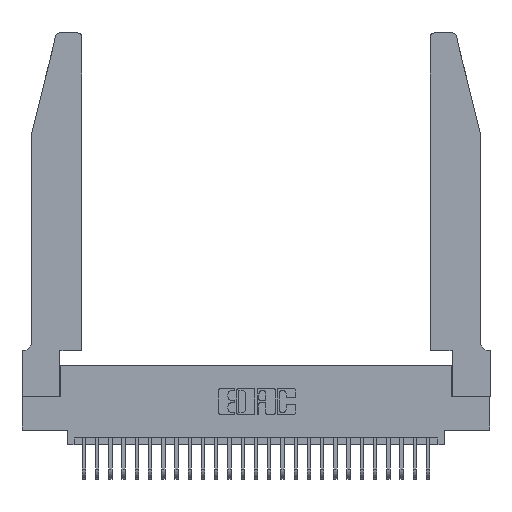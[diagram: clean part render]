
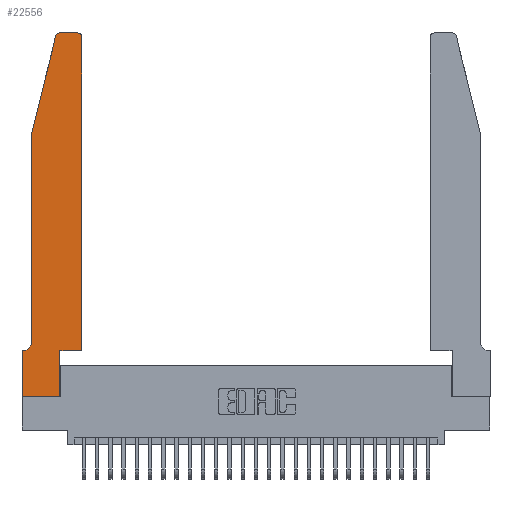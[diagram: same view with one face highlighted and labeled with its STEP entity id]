
A CAD part, top view. The second image highlights one B-rep face of the part: STEP entity #22556.
In plain terms, the highlighted planar face has unit normal (0, 0, 1).
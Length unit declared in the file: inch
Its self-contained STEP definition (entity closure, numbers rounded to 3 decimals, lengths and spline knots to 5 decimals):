
#375 = ORIENTED_EDGE ( 'NONE', *, *, #16951, .T. ) ;
#430 = CARTESIAN_POINT ( 'NONE',  ( 0.4505, 0.35, 0.37 ) ) ;
#533 = ORIENTED_EDGE ( 'NONE', *, *, #11669, .T. ) ;
#1488 = VECTOR ( 'NONE', #29293, 39.37008 ) ;
#1646 = VECTOR ( 'NONE', #20844, 39.37008 ) ;
#1717 = EDGE_CURVE ( 'NONE', #22528, #5723, #22442, .T. ) ;
#1726 = AXIS2_PLACEMENT_3D ( 'NONE', #11985, #23488, #21390 ) ;
#1741 = ORIENTED_EDGE ( 'NONE', *, *, #27079, .T. ) ;
#1800 = CARTESIAN_POINT ( 'NONE',  ( 0., 0., 0.37 ) ) ;
#2905 = CARTESIAN_POINT ( 'NONE',  ( 0.4505, 0.35, 0.37 ) ) ;
#2944 = CARTESIAN_POINT ( 'NONE',  ( 0.0055, 0.35, 0.37 ) ) ;
#3498 = CARTESIAN_POINT ( 'NONE',  ( 0., 0., 0.37 ) ) ;
#3584 = ORIENTED_EDGE ( 'NONE', *, *, #4587, .T. ) ;
#4185 = LINE ( 'NONE', #24555, #15647 ) ;
#4266 = DIRECTION ( 'NONE',  ( -1., 0., 0. ) ) ;
#4587 = EDGE_CURVE ( 'NONE', #23105, #7640, #13670, .T. ) ;
#4947 = CARTESIAN_POINT ( 'NONE',  ( 0.0755, 0.42, 0.37 ) ) ;
#5068 = VERTEX_POINT ( 'NONE', #10028 ) ;
#5439 = VECTOR ( 'NONE', #25315, 39.37008 ) ;
#5459 = ORIENTED_EDGE ( 'NONE', *, *, #1717, .T. ) ;
#5581 = FACE_OUTER_BOUND ( 'NONE', #8684, .T. ) ;
#5723 = VERTEX_POINT ( 'NONE', #19991 ) ;
#6921 = DIRECTION ( 'NONE',  ( 0., -1., 0. ) ) ;
#6987 = ORIENTED_EDGE ( 'NONE', *, *, #10676, .T. ) ;
#7568 = ORIENTED_EDGE ( 'NONE', *, *, #29201, .T. ) ;
#7640 = VERTEX_POINT ( 'NONE', #20944 ) ;
#7680 = CARTESIAN_POINT ( 'NONE',  ( 0.2865, 0.35, 0.37 ) ) ;
#8175 = CARTESIAN_POINT ( 'NONE',  ( 0.4205, 2.75, 0.37 ) ) ;
#8197 = LINE ( 'NONE', #2905, #18227 ) ;
#8434 = LINE ( 'NONE', #11802, #26037 ) ;
#8684 = EDGE_LOOP ( 'NONE', ( #5459, #12279, #17087, #6987, #375, #15100, #533, #3584, #7568, #1741, #19392, #16044 ) ) ;
#9358 = DIRECTION ( 'NONE',  ( 1., 0., 0. ) ) ;
#10028 = CARTESIAN_POINT ( 'NONE',  ( 0.0755, 2., 0.37 ) ) ;
#10676 = EDGE_CURVE ( 'NONE', #5068, #27703, #4185, .T. ) ;
#10767 = CARTESIAN_POINT ( 'NONE',  ( 0.4205, 2.72, 0.37 ) ) ;
#11491 = CARTESIAN_POINT ( 'NONE',  ( 0.4505, 2.72, 0.37 ) ) ;
#11669 = EDGE_CURVE ( 'NONE', #23673, #23105, #23116, .T. ) ;
#11802 = CARTESIAN_POINT ( 'NONE',  ( 0.2865, 0.35, 0.37 ) ) ;
#11940 = DIRECTION ( 'NONE',  ( 0., 0., 1. ) ) ;
#11985 = CARTESIAN_POINT ( 'NONE',  ( 0.0055, 0.42, 0.37 ) ) ;
#12279 = ORIENTED_EDGE ( 'NONE', *, *, #28305, .T. ) ;
#12955 = VECTOR ( 'NONE', #21468, 39.37008 ) ;
#13012 = DIRECTION ( 'NONE',  ( 1., 0., 0. ) ) ;
#13096 = AXIS2_PLACEMENT_3D ( 'NONE', #10767, #27358, #29496 ) ;
#13130 = EDGE_CURVE ( 'NONE', #19596, #28972, #14372, .T. ) ;
#13670 = LINE ( 'NONE', #25472, #12955 ) ;
#14372 = LINE ( 'NONE', #24718, #1488 ) ;
#14900 = DIRECTION ( 'NONE',  ( 0., 0., 1. ) ) ;
#15100 = ORIENTED_EDGE ( 'NONE', *, *, #19973, .T. ) ;
#15647 = VECTOR ( 'NONE', #6921, 39.37008 ) ;
#16044 = ORIENTED_EDGE ( 'NONE', *, *, #19439, .T. ) ;
#16383 = DIRECTION ( 'NONE',  ( 0., 1., 0. ) ) ;
#16781 = CIRCLE ( 'NONE', #13096, 0.03 ) ;
#16951 = EDGE_CURVE ( 'NONE', #27703, #26474, #25640, .T. ) ;
#17087 = ORIENTED_EDGE ( 'NONE', *, *, #24657, .T. ) ;
#17845 = CARTESIAN_POINT ( 'NONE',  ( 0.0755, 0.35, 0.37 ) ) ;
#17927 = LINE ( 'NONE', #22639, #5439 ) ;
#18227 = VECTOR ( 'NONE', #9358, 39.37008 ) ;
#19392 = ORIENTED_EDGE ( 'NONE', *, *, #13130, .T. ) ;
#19439 = EDGE_CURVE ( 'NONE', #28972, #22528, #16781, .T. ) ;
#19596 = VERTEX_POINT ( 'NONE', #430 ) ;
#19973 = EDGE_CURVE ( 'NONE', #26474, #23673, #25398, .T. ) ;
#19991 = CARTESIAN_POINT ( 'NONE',  ( 0.284, 2.75, 0.37 ) ) ;
#20844 = DIRECTION ( 'NONE',  ( -1., 0., 0. ) ) ;
#20944 = CARTESIAN_POINT ( 'NONE',  ( 0.2865, 0., 0.37 ) ) ;
#21280 = AXIS2_PLACEMENT_3D ( 'NONE', #23348, #11940, #21352 ) ;
#21352 = DIRECTION ( 'NONE',  ( 1., 0., 0. ) ) ;
#21390 = DIRECTION ( 'NONE',  ( -1., 0., 0. ) ) ;
#21468 = DIRECTION ( 'NONE',  ( 1., 0., 0. ) ) ;
#22027 = CARTESIAN_POINT ( 'NONE',  ( 0., 0.35, 0.37 ) ) ;
#22442 = LINE ( 'NONE', #23070, #1646 ) ;
#22528 = VERTEX_POINT ( 'NONE', #8175 ) ;
#22556 = ADVANCED_FACE ( 'NONE', ( #5581 ), #24220, .T. ) ;
#22639 = CARTESIAN_POINT ( 'NONE',  ( 0.0755, 2., 0.37 ) ) ;
#23070 = CARTESIAN_POINT ( 'NONE',  ( 0.2605, 2.75, 0.37 ) ) ;
#23105 = VERTEX_POINT ( 'NONE', #3498 ) ;
#23116 = LINE ( 'NONE', #1800, #28542 ) ;
#23348 = CARTESIAN_POINT ( 'NONE',  ( 0.284, 2.72, 0.37 ) ) ;
#23488 = DIRECTION ( 'NONE',  ( 0., 0., -1. ) ) ;
#23673 = VERTEX_POINT ( 'NONE', #23969 ) ;
#23969 = CARTESIAN_POINT ( 'NONE',  ( 0., 0.35, 0.37 ) ) ;
#24220 = PLANE ( 'NONE',  #29508 ) ;
#24555 = CARTESIAN_POINT ( 'NONE',  ( 0.0755, 2., 0.37 ) ) ;
#24657 = EDGE_CURVE ( 'NONE', #27286, #5068, #17927, .T. ) ;
#24718 = CARTESIAN_POINT ( 'NONE',  ( 0.4505, 0.35, 0.37 ) ) ;
#25033 = VECTOR ( 'NONE', #4266, 39.37008 ) ;
#25315 = DIRECTION ( 'NONE',  ( -0.239, -0.971, 0. ) ) ;
#25351 = CIRCLE ( 'NONE', #21280, 0.03 ) ;
#25398 = LINE ( 'NONE', #17845, #25033 ) ;
#25472 = CARTESIAN_POINT ( 'NONE',  ( 0., 0., 0.37 ) ) ;
#25640 = CIRCLE ( 'NONE', #1726, 0.07 ) ;
#26037 = VECTOR ( 'NONE', #16383, 39.37008 ) ;
#26474 = VERTEX_POINT ( 'NONE', #2944 ) ;
#26863 = DIRECTION ( 'NONE',  ( 0., -1., 0. ) ) ;
#27079 = EDGE_CURVE ( 'NONE', #27221, #19596, #8197, .T. ) ;
#27221 = VERTEX_POINT ( 'NONE', #7680 ) ;
#27286 = VERTEX_POINT ( 'NONE', #28956 ) ;
#27358 = DIRECTION ( 'NONE',  ( 0., 0., 1. ) ) ;
#27703 = VERTEX_POINT ( 'NONE', #4947 ) ;
#28305 = EDGE_CURVE ( 'NONE', #5723, #27286, #25351, .T. ) ;
#28542 = VECTOR ( 'NONE', #26863, 39.37008 ) ;
#28956 = CARTESIAN_POINT ( 'NONE',  ( 0.25487, 2.72718, 0.37 ) ) ;
#28972 = VERTEX_POINT ( 'NONE', #11491 ) ;
#29201 = EDGE_CURVE ( 'NONE', #7640, #27221, #8434, .T. ) ;
#29293 = DIRECTION ( 'NONE',  ( 0., 1., 0. ) ) ;
#29496 = DIRECTION ( 'NONE',  ( 1., 0., 0. ) ) ;
#29508 = AXIS2_PLACEMENT_3D ( 'NONE', #22027, #14900, #13012 ) ;
